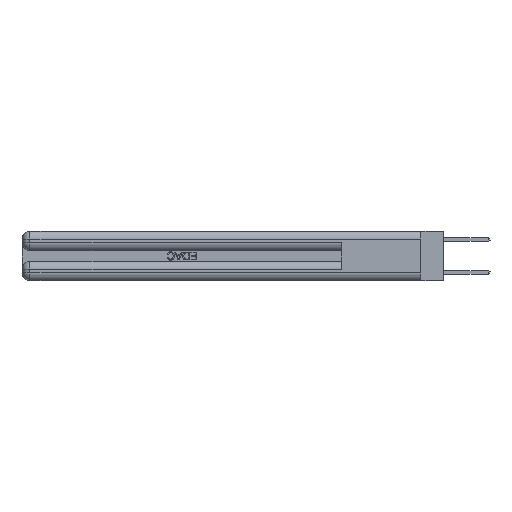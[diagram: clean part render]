
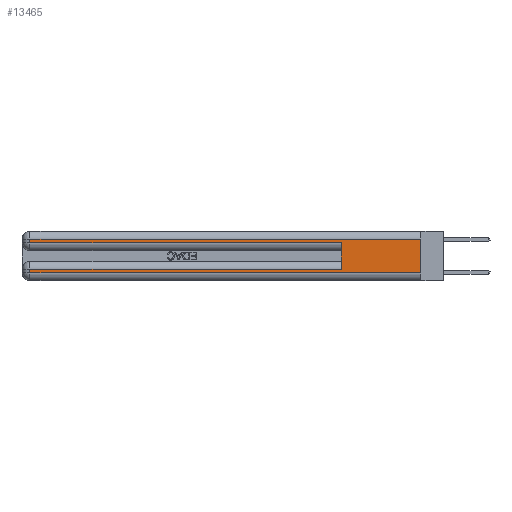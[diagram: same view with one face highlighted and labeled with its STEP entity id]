
A CAD part, left-side view. The second image highlights one B-rep face of the part: STEP entity #13465.
In plain terms, the highlighted planar face has unit normal (-1, 0, 0).
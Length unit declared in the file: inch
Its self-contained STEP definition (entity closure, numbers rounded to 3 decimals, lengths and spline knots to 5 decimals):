
#441 = VECTOR ( 'NONE', #7730, 39.37008 ) ;
#493 = DIRECTION ( 'NONE',  ( 0., 0., 1. ) ) ;
#867 = DIRECTION ( 'NONE',  ( 1., 0., 0. ) ) ;
#987 = DIRECTION ( 'NONE',  ( 0., 0., -1. ) ) ;
#1057 = VERTEX_POINT ( 'NONE', #16621 ) ;
#1116 = LINE ( 'NONE', #14377, #4850 ) ;
#1311 = CARTESIAN_POINT ( 'NONE',  ( 0., 0., 0.37 ) ) ;
#1867 = VECTOR ( 'NONE', #12234, 39.37008 ) ;
#2165 = EDGE_CURVE ( 'NONE', #22784, #5657, #12451, .T. ) ;
#2721 = EDGE_CURVE ( 'NONE', #7253, #5657, #15597, .T. ) ;
#2929 = VECTOR ( 'NONE', #493, 39.37008 ) ;
#3364 = EDGE_LOOP ( 'NONE', ( #21279, #29491, #30533, #13666, #24800, #7949, #23994, #32566 ) ) ;
#4512 = LINE ( 'NONE', #25028, #1867 ) ;
#4850 = VECTOR ( 'NONE', #31720, 39.37008 ) ;
#5657 = VERTEX_POINT ( 'NONE', #23903 ) ;
#7083 = LINE ( 'NONE', #20362, #26404 ) ;
#7253 = VERTEX_POINT ( 'NONE', #7441 ) ;
#7441 = CARTESIAN_POINT ( 'NONE',  ( 0., 0.6, 0.085 ) ) ;
#7543 = VERTEX_POINT ( 'NONE', #10372 ) ;
#7730 = DIRECTION ( 'NONE',  ( 0., -1., 0. ) ) ;
#7949 = ORIENTED_EDGE ( 'NONE', *, *, #15964, .T. ) ;
#8573 = CARTESIAN_POINT ( 'NONE',  ( 0., 2.94, 0.285 ) ) ;
#9598 = VECTOR ( 'NONE', #987, 39.37008 ) ;
#10372 = CARTESIAN_POINT ( 'NONE',  ( 0., 0., 0.31 ) ) ;
#11097 = DIRECTION ( 'NONE',  ( 0., 0., -1. ) ) ;
#11704 = LINE ( 'NONE', #1311, #9598 ) ;
#11739 = DIRECTION ( 'NONE',  ( 0., 1., 0. ) ) ;
#12234 = DIRECTION ( 'NONE',  ( 0., 0., -1. ) ) ;
#12451 = LINE ( 'NONE', #32977, #441 ) ;
#12621 = VERTEX_POINT ( 'NONE', #25498 ) ;
#13307 = VECTOR ( 'NONE', #11739, 39.37008 ) ;
#13465 = ADVANCED_FACE ( 'NONE', ( #13615 ), #25913, .F. ) ;
#13528 = DIRECTION ( 'NONE',  ( 0., -1., 0. ) ) ;
#13615 = FACE_OUTER_BOUND ( 'NONE', #3364, .T. ) ;
#13666 = ORIENTED_EDGE ( 'NONE', *, *, #2165, .T. ) ;
#14377 = CARTESIAN_POINT ( 'NONE',  ( 0., 2.94, 0.37 ) ) ;
#14603 = LINE ( 'NONE', #19804, #13307 ) ;
#15597 = LINE ( 'NONE', #23339, #2929 ) ;
#15964 = EDGE_CURVE ( 'NONE', #7253, #27748, #14603, .T. ) ;
#16252 = CARTESIAN_POINT ( 'NONE',  ( 0., 2.94, 0.31 ) ) ;
#16621 = CARTESIAN_POINT ( 'NONE',  ( 0., 0., 0.06 ) ) ;
#17330 = EDGE_CURVE ( 'NONE', #7543, #1057, #11704, .T. ) ;
#17338 = DIRECTION ( 'NONE',  ( 0., 1., 0. ) ) ;
#18807 = EDGE_CURVE ( 'NONE', #27748, #12621, #1116, .T. ) ;
#19804 = CARTESIAN_POINT ( 'NONE',  ( 0., 0., 0.085 ) ) ;
#20254 = EDGE_CURVE ( 'NONE', #12621, #1057, #26330, .T. ) ;
#20362 = CARTESIAN_POINT ( 'NONE',  ( 0., 0., 0.31 ) ) ;
#20999 = CARTESIAN_POINT ( 'NONE',  ( 0., 2.94, 0.085 ) ) ;
#21279 = ORIENTED_EDGE ( 'NONE', *, *, #17330, .F. ) ;
#22479 = EDGE_CURVE ( 'NONE', #7543, #30684, #7083, .T. ) ;
#22784 = VERTEX_POINT ( 'NONE', #8573 ) ;
#23339 = CARTESIAN_POINT ( 'NONE',  ( 0., 0.6, 0.145 ) ) ;
#23874 = CARTESIAN_POINT ( 'NONE',  ( 0., 0., 0.37 ) ) ;
#23903 = CARTESIAN_POINT ( 'NONE',  ( 0., 0.6, 0.285 ) ) ;
#23994 = ORIENTED_EDGE ( 'NONE', *, *, #18807, .T. ) ;
#24800 = ORIENTED_EDGE ( 'NONE', *, *, #2721, .F. ) ;
#25028 = CARTESIAN_POINT ( 'NONE',  ( 0., 2.94, 0.37 ) ) ;
#25498 = CARTESIAN_POINT ( 'NONE',  ( 0., 2.94, 0.06 ) ) ;
#25913 = PLANE ( 'NONE',  #31995 ) ;
#26330 = LINE ( 'NONE', #31212, #29030 ) ;
#26404 = VECTOR ( 'NONE', #17338, 39.37008 ) ;
#27748 = VERTEX_POINT ( 'NONE', #20999 ) ;
#29030 = VECTOR ( 'NONE', #13528, 39.37008 ) ;
#29491 = ORIENTED_EDGE ( 'NONE', *, *, #22479, .T. ) ;
#30376 = EDGE_CURVE ( 'NONE', #30684, #22784, #4512, .T. ) ;
#30533 = ORIENTED_EDGE ( 'NONE', *, *, #30376, .T. ) ;
#30684 = VERTEX_POINT ( 'NONE', #16252 ) ;
#31212 = CARTESIAN_POINT ( 'NONE',  ( 0., 0., 0.06 ) ) ;
#31720 = DIRECTION ( 'NONE',  ( 0., 0., -1. ) ) ;
#31995 = AXIS2_PLACEMENT_3D ( 'NONE', #23874, #867, #11097 ) ;
#32566 = ORIENTED_EDGE ( 'NONE', *, *, #20254, .T. ) ;
#32977 = CARTESIAN_POINT ( 'NONE',  ( 0., 0., 0.285 ) ) ;
